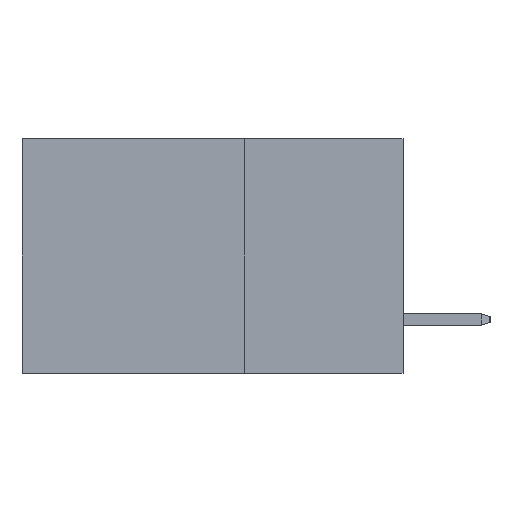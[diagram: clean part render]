
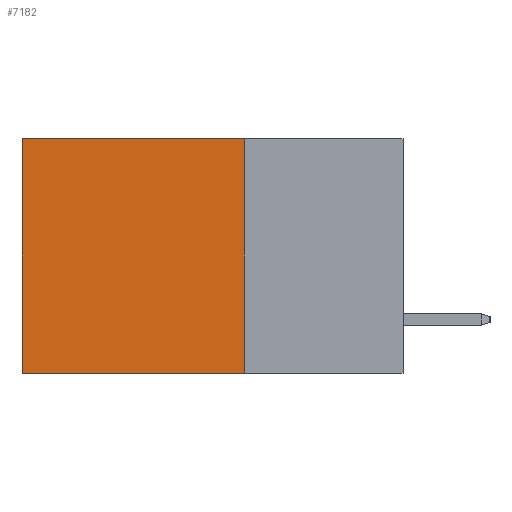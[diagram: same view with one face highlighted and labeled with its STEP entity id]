
A CAD part, left-side view. The second image highlights one B-rep face of the part: STEP entity #7182.
In plain terms, the highlighted planar face has unit normal (-1, 0, 0).
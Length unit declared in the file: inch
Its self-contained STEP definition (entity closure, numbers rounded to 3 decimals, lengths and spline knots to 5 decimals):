
#51 = LINE ( 'NONE', #13296, #4555 ) ;
#194 = DIRECTION ( 'NONE',  ( 0., 0., -1. ) ) ;
#1155 = VECTOR ( 'NONE', #7761, 39.37008 ) ;
#2630 = DIRECTION ( 'NONE',  ( 0., 0., -1. ) ) ;
#2754 = CARTESIAN_POINT ( 'NONE',  ( 0.2875, 0.6, 0. ) ) ;
#2948 = ORIENTED_EDGE ( 'NONE', *, *, #12852, .F. ) ;
#4555 = VECTOR ( 'NONE', #9694, 39.37008 ) ;
#5109 = CARTESIAN_POINT ( 'NONE',  ( 0.2875, 0.25, 0. ) ) ;
#5641 = VERTEX_POINT ( 'NONE', #10080 ) ;
#5819 = ORIENTED_EDGE ( 'NONE', *, *, #12322, .T. ) ;
#5857 = ORIENTED_EDGE ( 'NONE', *, *, #6508, .T. ) ;
#5917 = CARTESIAN_POINT ( 'NONE',  ( 0.2875, 0.25, -0.37 ) ) ;
#6101 = LINE ( 'NONE', #10937, #10513 ) ;
#6123 = VECTOR ( 'NONE', #8825, 39.37008 ) ;
#6508 = EDGE_CURVE ( 'NONE', #9505, #5641, #7563, .T. ) ;
#7182 = ADVANCED_FACE ( 'NONE', ( #7624 ), #7469, .F. ) ;
#7396 = DIRECTION ( 'NONE',  ( 1., 0., 0. ) ) ;
#7469 = PLANE ( 'NONE',  #14513 ) ;
#7563 = LINE ( 'NONE', #11028, #6123 ) ;
#7624 = FACE_OUTER_BOUND ( 'NONE', #11680, .T. ) ;
#7713 = EDGE_CURVE ( 'NONE', #7938, #5641, #8866, .T. ) ;
#7761 = DIRECTION ( 'NONE',  ( 0., 1., 0. ) ) ;
#7938 = VERTEX_POINT ( 'NONE', #5917 ) ;
#8825 = DIRECTION ( 'NONE',  ( 0., 0., -1. ) ) ;
#8866 = LINE ( 'NONE', #11453, #1155 ) ;
#9388 = ORIENTED_EDGE ( 'NONE', *, *, #7713, .F. ) ;
#9505 = VERTEX_POINT ( 'NONE', #2754 ) ;
#9694 = DIRECTION ( 'NONE',  ( 0., 1., 0. ) ) ;
#10080 = CARTESIAN_POINT ( 'NONE',  ( 0.2875, 0.6, -0.37 ) ) ;
#10513 = VECTOR ( 'NONE', #2630, 39.37008 ) ;
#10937 = CARTESIAN_POINT ( 'NONE',  ( 0.2875, 0.25, 0. ) ) ;
#10941 = CARTESIAN_POINT ( 'NONE',  ( 0.2875, 0.25, 0. ) ) ;
#11028 = CARTESIAN_POINT ( 'NONE',  ( 0.2875, 0.6, 0. ) ) ;
#11453 = CARTESIAN_POINT ( 'NONE',  ( 0.2875, 0.25, -0.37 ) ) ;
#11680 = EDGE_LOOP ( 'NONE', ( #5857, #9388, #2948, #5819 ) ) ;
#12322 = EDGE_CURVE ( 'NONE', #15092, #9505, #51, .T. ) ;
#12852 = EDGE_CURVE ( 'NONE', #15092, #7938, #6101, .T. ) ;
#13296 = CARTESIAN_POINT ( 'NONE',  ( 0.2875, 0.25, 0. ) ) ;
#14513 = AXIS2_PLACEMENT_3D ( 'NONE', #10941, #7396, #194 ) ;
#15092 = VERTEX_POINT ( 'NONE', #5109 ) ;
